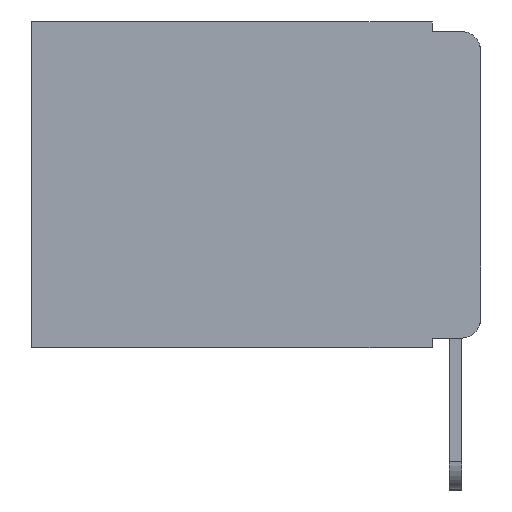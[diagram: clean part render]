
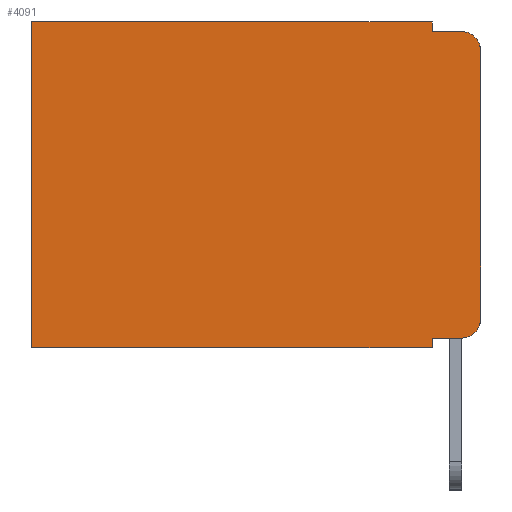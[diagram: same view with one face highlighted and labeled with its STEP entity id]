
A CAD part, left-side view. The second image highlights one B-rep face of the part: STEP entity #4091.
In plain terms, the highlighted planar face has unit normal (-1, 0, 0).
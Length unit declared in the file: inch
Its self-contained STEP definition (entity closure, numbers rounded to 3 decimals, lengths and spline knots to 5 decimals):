
#102 = VERTEX_POINT ( 'NONE', #5220 ) ;
#227 = LINE ( 'NONE', #6304, #7078 ) ;
#415 = VECTOR ( 'NONE', #13017, 39.37008 ) ;
#653 = CIRCLE ( 'NONE', #4850, 0.02 ) ;
#990 = DIRECTION ( 'NONE',  ( 0., 0., -1. ) ) ;
#2069 = LINE ( 'NONE', #7313, #13801 ) ;
#2296 = DIRECTION ( 'NONE',  ( 0., 1., 0. ) ) ;
#2297 = CARTESIAN_POINT ( 'NONE',  ( 0.298, 0.473, 0. ) ) ;
#2400 = DIRECTION ( 'NONE',  ( 0., 0., -1. ) ) ;
#2559 = CARTESIAN_POINT ( 'NONE',  ( 0.298, 0.473, 0. ) ) ;
#2695 = CIRCLE ( 'NONE', #8180, 0.02 ) ;
#3142 = DIRECTION ( 'NONE',  ( 0., 1., 0. ) ) ;
#3204 = CARTESIAN_POINT ( 'NONE',  ( 0.298, 0.02, -0.03 ) ) ;
#3392 = LINE ( 'NONE', #9369, #15132 ) ;
#3669 = DIRECTION ( 'NONE',  ( 0., 0., -1. ) ) ;
#3801 = CARTESIAN_POINT ( 'NONE',  ( 0.298, 0.051, 0. ) ) ;
#4091 = ADVANCED_FACE ( 'NONE', ( #4634 ), #7390, .F. ) ;
#4209 = CARTESIAN_POINT ( 'NONE',  ( 0.298, 0., 0. ) ) ;
#4401 = LINE ( 'NONE', #13414, #7400 ) ;
#4563 = DIRECTION ( 'NONE',  ( 0., 0., -1. ) ) ;
#4634 = FACE_OUTER_BOUND ( 'NONE', #7031, .T. ) ;
#4796 = DIRECTION ( 'NONE',  ( -1., 0., 0. ) ) ;
#4850 = AXIS2_PLACEMENT_3D ( 'NONE', #3204, #11479, #4563 ) ;
#5147 = CARTESIAN_POINT ( 'NONE',  ( 0.298, 0.051, 0. ) ) ;
#5204 = VERTEX_POINT ( 'NONE', #9973 ) ;
#5220 = CARTESIAN_POINT ( 'NONE',  ( 0.298, 0.051, -0.01 ) ) ;
#5378 = VERTEX_POINT ( 'NONE', #13555 ) ;
#5395 = VERTEX_POINT ( 'NONE', #9462 ) ;
#5537 = LINE ( 'NONE', #5147, #10891 ) ;
#5589 = EDGE_CURVE ( 'NONE', #6798, #102, #5537, .T. ) ;
#6304 = CARTESIAN_POINT ( 'NONE',  ( 0.298, 0., -0.343 ) ) ;
#6426 = EDGE_CURVE ( 'NONE', #10395, #6994, #9046, .T. ) ;
#6703 = DIRECTION ( 'NONE',  ( 0., -1., 0. ) ) ;
#6798 = VERTEX_POINT ( 'NONE', #7245 ) ;
#6994 = VERTEX_POINT ( 'NONE', #11855 ) ;
#7031 = EDGE_LOOP ( 'NONE', ( #14273, #14391, #14438, #14455, #14483, #14722, #14761, #14793, #14848, #15020 ) ) ;
#7078 = VECTOR ( 'NONE', #2296, 39.37008 ) ;
#7245 = CARTESIAN_POINT ( 'NONE',  ( 0.298, 0.051, 0. ) ) ;
#7313 = CARTESIAN_POINT ( 'NONE',  ( 0.298, 0.051, -0.333 ) ) ;
#7318 = VERTEX_POINT ( 'NONE', #10262 ) ;
#7359 = CARTESIAN_POINT ( 'NONE',  ( 0.298, 0.02, -0.01 ) ) ;
#7390 = PLANE ( 'NONE',  #11922 ) ;
#7400 = VECTOR ( 'NONE', #8094, 39.37008 ) ;
#7445 = EDGE_CURVE ( 'NONE', #6798, #10395, #3392, .T. ) ;
#7607 = EDGE_CURVE ( 'NONE', #7698, #5378, #2069, .T. ) ;
#7616 = VECTOR ( 'NONE', #6703, 39.37008 ) ;
#7698 = VERTEX_POINT ( 'NONE', #13835 ) ;
#7770 = EDGE_CURVE ( 'NONE', #5204, #6994, #227, .T. ) ;
#8094 = DIRECTION ( 'NONE',  ( 0., 0., -1. ) ) ;
#8180 = AXIS2_PLACEMENT_3D ( 'NONE', #11659, #4796, #12723 ) ;
#8992 = CARTESIAN_POINT ( 'NONE',  ( 0.298, 0.051, -0.01 ) ) ;
#9046 = LINE ( 'NONE', #2297, #14288 ) ;
#9146 = VERTEX_POINT ( 'NONE', #7359 ) ;
#9244 = EDGE_CURVE ( 'NONE', #7698, #5204, #12978, .T. ) ;
#9369 = CARTESIAN_POINT ( 'NONE',  ( 0.298, 0., 0. ) ) ;
#9462 = CARTESIAN_POINT ( 'NONE',  ( 0.298, 0., -0.03 ) ) ;
#9469 = EDGE_CURVE ( 'NONE', #5395, #7318, #4401, .T. ) ;
#9602 = DIRECTION ( 'NONE',  ( 0., -1., 0. ) ) ;
#9779 = DIRECTION ( 'NONE',  ( 1., 0., 0. ) ) ;
#9973 = CARTESIAN_POINT ( 'NONE',  ( 0.298, 0.051, -0.343 ) ) ;
#10262 = CARTESIAN_POINT ( 'NONE',  ( 0.298, 0., -0.313 ) ) ;
#10395 = VERTEX_POINT ( 'NONE', #2559 ) ;
#10891 = VECTOR ( 'NONE', #990, 39.37008 ) ;
#11479 = DIRECTION ( 'NONE',  ( -1., 0., 0. ) ) ;
#11659 = CARTESIAN_POINT ( 'NONE',  ( 0.298, 0.02, -0.313 ) ) ;
#11855 = CARTESIAN_POINT ( 'NONE',  ( 0.298, 0.473, -0.343 ) ) ;
#11922 = AXIS2_PLACEMENT_3D ( 'NONE', #4209, #9779, #2400 ) ;
#12723 = DIRECTION ( 'NONE',  ( 0., 0., -1. ) ) ;
#12978 = LINE ( 'NONE', #3801, #415 ) ;
#13017 = DIRECTION ( 'NONE',  ( 0., 0., -1. ) ) ;
#13048 = EDGE_CURVE ( 'NONE', #102, #9146, #13640, .T. ) ;
#13414 = CARTESIAN_POINT ( 'NONE',  ( 0.298, 0., 0. ) ) ;
#13427 = EDGE_CURVE ( 'NONE', #5395, #9146, #653, .T. ) ;
#13555 = CARTESIAN_POINT ( 'NONE',  ( 0.298, 0.02, -0.333 ) ) ;
#13627 = EDGE_CURVE ( 'NONE', #5378, #7318, #2695, .T. ) ;
#13640 = LINE ( 'NONE', #8992, #7616 ) ;
#13801 = VECTOR ( 'NONE', #9602, 39.37008 ) ;
#13835 = CARTESIAN_POINT ( 'NONE',  ( 0.298, 0.051, -0.333 ) ) ;
#14273 = ORIENTED_EDGE ( 'NONE', *, *, #9469, .F. ) ;
#14288 = VECTOR ( 'NONE', #3669, 39.37008 ) ;
#14391 = ORIENTED_EDGE ( 'NONE', *, *, #13427, .T. ) ;
#14438 = ORIENTED_EDGE ( 'NONE', *, *, #13048, .F. ) ;
#14455 = ORIENTED_EDGE ( 'NONE', *, *, #5589, .F. ) ;
#14483 = ORIENTED_EDGE ( 'NONE', *, *, #7445, .T. ) ;
#14722 = ORIENTED_EDGE ( 'NONE', *, *, #6426, .T. ) ;
#14761 = ORIENTED_EDGE ( 'NONE', *, *, #7770, .F. ) ;
#14793 = ORIENTED_EDGE ( 'NONE', *, *, #9244, .F. ) ;
#14848 = ORIENTED_EDGE ( 'NONE', *, *, #7607, .T. ) ;
#15020 = ORIENTED_EDGE ( 'NONE', *, *, #13627, .T. ) ;
#15132 = VECTOR ( 'NONE', #3142, 39.37008 ) ;
